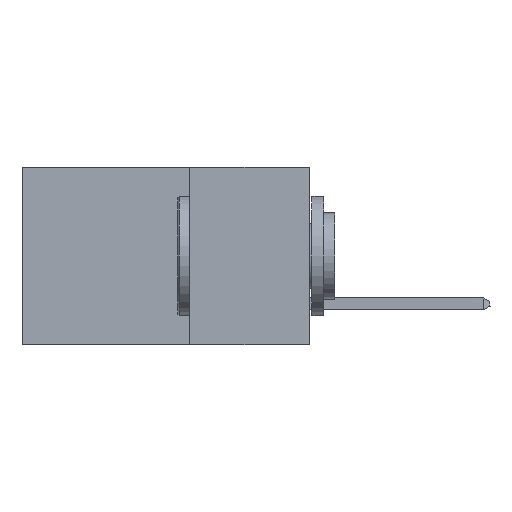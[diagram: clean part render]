
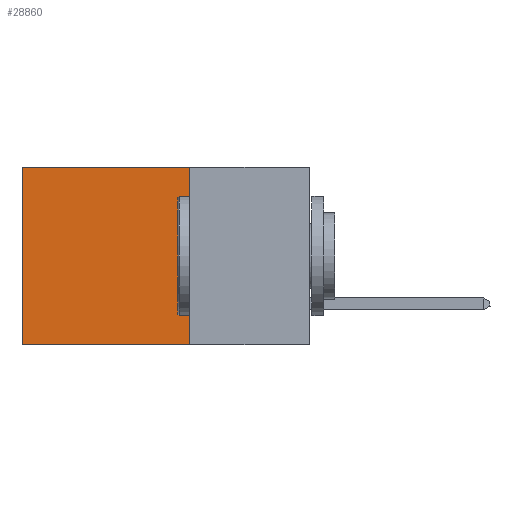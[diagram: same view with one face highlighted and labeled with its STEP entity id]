
A CAD part, left-side view. The second image highlights one B-rep face of the part: STEP entity #28860.
In plain terms, the highlighted planar face has unit normal (-1, 0, 0).
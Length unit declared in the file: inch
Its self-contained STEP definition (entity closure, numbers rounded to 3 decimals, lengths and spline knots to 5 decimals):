
#1000 = EDGE_LOOP ( 'NONE', ( #33009, #17836, #11847, #45290 ) ) ;
#1209 = LINE ( 'NONE', #2985, #17734 ) ;
#2985 = CARTESIAN_POINT ( 'NONE',  ( 0.2875, 0.25, -0.37 ) ) ;
#4030 = DIRECTION ( 'NONE',  ( 0., 0., -1. ) ) ;
#4632 = CARTESIAN_POINT ( 'NONE',  ( 0.2875, 0.25, 0. ) ) ;
#6228 = VERTEX_POINT ( 'NONE', #46293 ) ;
#8644 = EDGE_CURVE ( 'NONE', #37297, #6228, #26969, .T. ) ;
#8717 = DIRECTION ( 'NONE',  ( 0., 1., 0. ) ) ;
#9136 = LINE ( 'NONE', #20118, #43177 ) ;
#11847 = ORIENTED_EDGE ( 'NONE', *, *, #8644, .F. ) ;
#14275 = CARTESIAN_POINT ( 'NONE',  ( 0.2875, 0.25, 0. ) ) ;
#15802 = CARTESIAN_POINT ( 'NONE',  ( 0.2875, 0.6, 0. ) ) ;
#17734 = VECTOR ( 'NONE', #45514, 39.37008 ) ;
#17836 = ORIENTED_EDGE ( 'NONE', *, *, #33414, .F. ) ;
#20118 = CARTESIAN_POINT ( 'NONE',  ( 0.2875, 0.25, 0. ) ) ;
#22631 = DIRECTION ( 'NONE',  ( 1., 0., 0. ) ) ;
#22809 = VERTEX_POINT ( 'NONE', #33015 ) ;
#23340 = AXIS2_PLACEMENT_3D ( 'NONE', #4632, #22631, #4030 ) ;
#23514 = EDGE_CURVE ( 'NONE', #22809, #46127, #24660, .T. ) ;
#24408 = VECTOR ( 'NONE', #40698, 39.37008 ) ;
#24660 = LINE ( 'NONE', #15802, #37455 ) ;
#26969 = LINE ( 'NONE', #14275, #24408 ) ;
#28860 = ADVANCED_FACE ( 'NONE', ( #44908 ), #39474, .F. ) ;
#29571 = DIRECTION ( 'NONE',  ( 0., 0., -1. ) ) ;
#31129 = CARTESIAN_POINT ( 'NONE',  ( 0.2875, 0.25, 0. ) ) ;
#33009 = ORIENTED_EDGE ( 'NONE', *, *, #23514, .T. ) ;
#33015 = CARTESIAN_POINT ( 'NONE',  ( 0.2875, 0.6, 0. ) ) ;
#33414 = EDGE_CURVE ( 'NONE', #6228, #46127, #1209, .T. ) ;
#37297 = VERTEX_POINT ( 'NONE', #31129 ) ;
#37455 = VECTOR ( 'NONE', #29571, 39.37008 ) ;
#39474 = PLANE ( 'NONE',  #23340 ) ;
#40698 = DIRECTION ( 'NONE',  ( 0., 0., -1. ) ) ;
#40902 = CARTESIAN_POINT ( 'NONE',  ( 0.2875, 0.6, -0.37 ) ) ;
#41840 = EDGE_CURVE ( 'NONE', #37297, #22809, #9136, .T. ) ;
#43177 = VECTOR ( 'NONE', #8717, 39.37008 ) ;
#44908 = FACE_OUTER_BOUND ( 'NONE', #1000, .T. ) ;
#45290 = ORIENTED_EDGE ( 'NONE', *, *, #41840, .T. ) ;
#45514 = DIRECTION ( 'NONE',  ( 0., 1., 0. ) ) ;
#46127 = VERTEX_POINT ( 'NONE', #40902 ) ;
#46293 = CARTESIAN_POINT ( 'NONE',  ( 0.2875, 0.25, -0.37 ) ) ;
